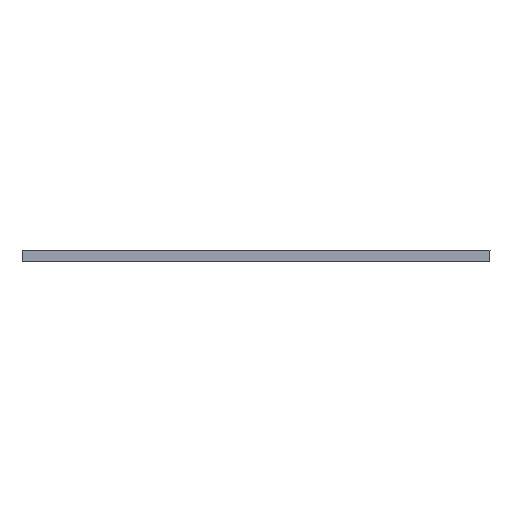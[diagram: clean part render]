
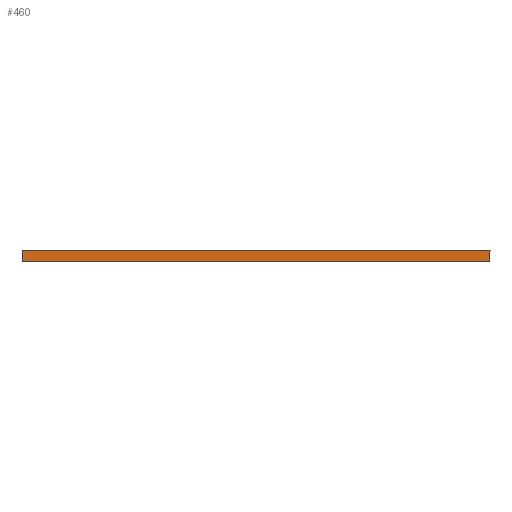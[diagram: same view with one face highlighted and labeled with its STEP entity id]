
A CAD part, left-side view. The second image highlights one B-rep face of the part: STEP entity #460.
In plain terms, the highlighted planar face has unit normal (-1, 0, 0).
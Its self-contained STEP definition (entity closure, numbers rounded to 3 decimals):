
#460 = ADVANCED_FACE ( 'NONE', ( #3234 ), #8940, .F. ) ;
#2184 = EDGE_CURVE ( 'NONE', #13751, #15239, #17650, .T. ) ;
#3234 = FACE_OUTER_BOUND ( 'NONE', #14902, .T. ) ;
#4006 = VERTEX_POINT ( 'NONE', #5499 ) ;
#4054 = EDGE_CURVE ( 'NONE', #4006, #15239, #7572, .T. ) ;
#5026 = CARTESIAN_POINT ( 'NONE',  ( -22.811, 20.5, 22.127 ) ) ;
#5499 = CARTESIAN_POINT ( 'NONE',  ( -22.811, -19.5, 22.127 ) ) ;
#5625 = DIRECTION ( 'NONE',  ( 0., -1., 0. ) ) ;
#5629 = CARTESIAN_POINT ( 'NONE',  ( -22.811, -19.5, 22.127 ) ) ;
#6601 = ORIENTED_EDGE ( 'NONE', *, *, #2184, .T. ) ;
#6940 = ORIENTED_EDGE ( 'NONE', *, *, #4054, .F. ) ;
#6984 = ORIENTED_EDGE ( 'NONE', *, *, #15310, .F. ) ;
#7092 = VECTOR ( 'NONE', #7110, 1000. ) ;
#7110 = DIRECTION ( 'NONE',  ( 0., 0., -1. ) ) ;
#7572 = LINE ( 'NONE', #5629, #7092 ) ;
#7778 = ORIENTED_EDGE ( 'NONE', *, *, #16386, .T. ) ;
#7817 = VERTEX_POINT ( 'NONE', #5026 ) ;
#8233 = CARTESIAN_POINT ( 'NONE',  ( -22.811, -19.5, 21.127 ) ) ;
#8346 = LINE ( 'NONE', #15706, #12175 ) ;
#8904 = CARTESIAN_POINT ( 'NONE',  ( -22.811, 20.5, 22.127 ) ) ;
#8940 = PLANE ( 'NONE',  #16273 ) ;
#9057 = DIRECTION ( 'NONE',  ( 1., 0., 0. ) ) ;
#9076 = DIRECTION ( 'NONE',  ( 0., 1., 0. ) ) ;
#10178 = VECTOR ( 'NONE', #10231, 1000. ) ;
#10231 = DIRECTION ( 'NONE',  ( 0., -1., 0. ) ) ;
#10825 = VECTOR ( 'NONE', #12826, 1000. ) ;
#11244 = LINE ( 'NONE', #11398, #10825 ) ;
#11398 = CARTESIAN_POINT ( 'NONE',  ( -22.811, 20.5, 22.127 ) ) ;
#11502 = CARTESIAN_POINT ( 'NONE',  ( -22.811, 20.5, 21.127 ) ) ;
#12175 = VECTOR ( 'NONE', #5625, 1000. ) ;
#12826 = DIRECTION ( 'NONE',  ( 0., 0., -1. ) ) ;
#13751 = VERTEX_POINT ( 'NONE', #16353 ) ;
#14902 = EDGE_LOOP ( 'NONE', ( #6601, #6940, #6984, #7778 ) ) ;
#15239 = VERTEX_POINT ( 'NONE', #8233 ) ;
#15310 = EDGE_CURVE ( 'NONE', #7817, #4006, #8346, .T. ) ;
#15706 = CARTESIAN_POINT ( 'NONE',  ( -22.811, 20.5, 22.127 ) ) ;
#16273 = AXIS2_PLACEMENT_3D ( 'NONE', #8904, #9057, #9076 ) ;
#16353 = CARTESIAN_POINT ( 'NONE',  ( -22.811, 20.5, 21.127 ) ) ;
#16386 = EDGE_CURVE ( 'NONE', #7817, #13751, #11244, .T. ) ;
#17650 = LINE ( 'NONE', #11502, #10178 ) ;
